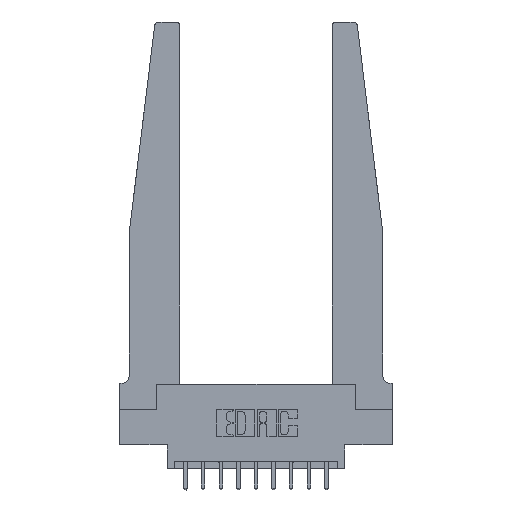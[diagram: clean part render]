
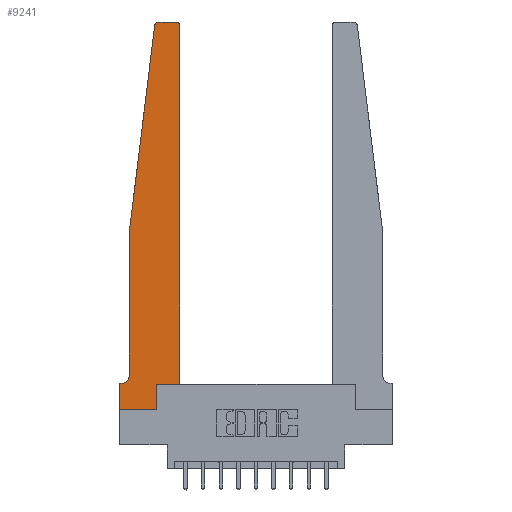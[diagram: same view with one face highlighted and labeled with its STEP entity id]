
A CAD part, top view. The second image highlights one B-rep face of the part: STEP entity #9241.
In plain terms, the highlighted planar face has unit normal (0, 0, 1).
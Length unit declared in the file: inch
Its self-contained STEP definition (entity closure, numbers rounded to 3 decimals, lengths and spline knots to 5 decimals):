
#208 = DIRECTION ( 'NONE',  ( -0.122, -0.992, 0. ) ) ;
#291 = DIRECTION ( 'NONE',  ( 0., 1., 0. ) ) ;
#334 = AXIS2_PLACEMENT_3D ( 'NONE', #9579, #2509, #10757 ) ;
#361 = VERTEX_POINT ( 'NONE', #12721 ) ;
#420 = CARTESIAN_POINT ( 'NONE',  ( 0.25, 2.75, 0.37 ) ) ;
#540 = CARTESIAN_POINT ( 'NONE',  ( 0.425, 0.18, 0.37 ) ) ;
#568 = EDGE_CURVE ( 'NONE', #1112, #13884, #9893, .T. ) ;
#876 = DIRECTION ( 'NONE',  ( 0., 0., 1. ) ) ;
#1070 = DIRECTION ( 'NONE',  ( -1., 0., 0. ) ) ;
#1112 = VERTEX_POINT ( 'NONE', #11998 ) ;
#1136 = CARTESIAN_POINT ( 'NONE',  ( 0., 0.1875, 0.37 ) ) ;
#1225 = EDGE_CURVE ( 'NONE', #2982, #15082, #8780, .T. ) ;
#1309 = ORIENTED_EDGE ( 'NONE', *, *, #10049, .T. ) ;
#1321 = CARTESIAN_POINT ( 'NONE',  ( 0.065, 0.1875, 0.37 ) ) ;
#1720 = AXIS2_PLACEMENT_3D ( 'NONE', #7896, #876, #9090 ) ;
#1835 = ORIENTED_EDGE ( 'NONE', *, *, #5461, .T. ) ;
#2044 = EDGE_CURVE ( 'NONE', #4084, #5762, #12457, .T. ) ;
#2156 = LINE ( 'NONE', #9585, #14345 ) ;
#2312 = CARTESIAN_POINT ( 'NONE',  ( 0.065, 1.25, 0.37 ) ) ;
#2509 = DIRECTION ( 'NONE',  ( 0., 0., 1. ) ) ;
#2982 = VERTEX_POINT ( 'NONE', #12450 ) ;
#3223 = CARTESIAN_POINT ( 'NONE',  ( 0.425, 0.18, 0.37 ) ) ;
#3772 = VECTOR ( 'NONE', #208, 39.37008 ) ;
#3892 = CIRCLE ( 'NONE', #6636, 0.03 ) ;
#4011 = AXIS2_PLACEMENT_3D ( 'NONE', #15167, #8103, #1070 ) ;
#4020 = VECTOR ( 'NONE', #7918, 39.37008 ) ;
#4084 = VERTEX_POINT ( 'NONE', #8564 ) ;
#4137 = CARTESIAN_POINT ( 'NONE',  ( 0.2605, 0.18, 0.37 ) ) ;
#4456 = ORIENTED_EDGE ( 'NONE', *, *, #14058, .T. ) ;
#4573 = EDGE_CURVE ( 'NONE', #7315, #1112, #5723, .T. ) ;
#4745 = ORIENTED_EDGE ( 'NONE', *, *, #12419, .T. ) ;
#5059 = EDGE_LOOP ( 'NONE', ( #5064, #1309, #12582, #4745, #6659, #11967, #1835, #11521, #14530, #4456, #9720, #8809 ) ) ;
#5064 = ORIENTED_EDGE ( 'NONE', *, *, #568, .T. ) ;
#5240 = EDGE_CURVE ( 'NONE', #5762, #14601, #10142, .T. ) ;
#5427 = CARTESIAN_POINT ( 'NONE',  ( 0.425, 2.72, 0.37 ) ) ;
#5461 = EDGE_CURVE ( 'NONE', #14601, #2982, #7173, .T. ) ;
#5523 = PLANE ( 'NONE',  #1720 ) ;
#5723 = CIRCLE ( 'NONE', #334, 0.03 ) ;
#5762 = VERTEX_POINT ( 'NONE', #8244 ) ;
#6111 = CARTESIAN_POINT ( 'NONE',  ( 0.425, 0.18, 0.37 ) ) ;
#6636 = AXIS2_PLACEMENT_3D ( 'NONE', #6956, #15228, #8160 ) ;
#6659 = ORIENTED_EDGE ( 'NONE', *, *, #2044, .T. ) ;
#6783 = DIRECTION ( 'NONE',  ( -1., 0., 0. ) ) ;
#6956 = CARTESIAN_POINT ( 'NONE',  ( 0.27653, 2.72, 0.37 ) ) ;
#6998 = VECTOR ( 'NONE', #9661, 39.37008 ) ;
#7074 = EDGE_CURVE ( 'NONE', #361, #13538, #13182, .T. ) ;
#7135 = LINE ( 'NONE', #3223, #4020 ) ;
#7173 = LINE ( 'NONE', #8831, #13088 ) ;
#7315 = VERTEX_POINT ( 'NONE', #5427 ) ;
#7667 = CARTESIAN_POINT ( 'NONE',  ( 0.27653, 2.75, 0.37 ) ) ;
#7896 = CARTESIAN_POINT ( 'NONE',  ( 0., 0.1875, 0.37 ) ) ;
#7918 = DIRECTION ( 'NONE',  ( 1., 0., 0. ) ) ;
#8030 = VECTOR ( 'NONE', #8179, 39.37008 ) ;
#8103 = DIRECTION ( 'NONE',  ( 0., 0., -1. ) ) ;
#8160 = DIRECTION ( 'NONE',  ( 1., 0., 0. ) ) ;
#8179 = DIRECTION ( 'NONE',  ( 1., 0., 0. ) ) ;
#8244 = CARTESIAN_POINT ( 'NONE',  ( 0.015, 0.1875, 0.37 ) ) ;
#8564 = CARTESIAN_POINT ( 'NONE',  ( 0.065, 0.2375, 0.37 ) ) ;
#8780 = LINE ( 'NONE', #11184, #8030 ) ;
#8809 = ORIENTED_EDGE ( 'NONE', *, *, #4573, .T. ) ;
#8831 = CARTESIAN_POINT ( 'NONE',  ( 0., 0., 0.37 ) ) ;
#8839 = VECTOR ( 'NONE', #291, 39.37008 ) ;
#9090 = DIRECTION ( 'NONE',  ( 1., 0., 0. ) ) ;
#9211 = LINE ( 'NONE', #6111, #8839 ) ;
#9241 = ADVANCED_FACE ( 'NONE', ( #12224 ), #5523, .T. ) ;
#9372 = CARTESIAN_POINT ( 'NONE',  ( 0.2605, 0.18, 0.37 ) ) ;
#9531 = VECTOR ( 'NONE', #6783, 39.37008 ) ;
#9579 = CARTESIAN_POINT ( 'NONE',  ( 0.395, 2.72, 0.37 ) ) ;
#9585 = CARTESIAN_POINT ( 'NONE',  ( 0.065, 1.25, 0.37 ) ) ;
#9661 = DIRECTION ( 'NONE',  ( -1., 0., 0. ) ) ;
#9720 = ORIENTED_EDGE ( 'NONE', *, *, #13704, .T. ) ;
#9763 = EDGE_CURVE ( 'NONE', #15082, #14181, #13858, .T. ) ;
#9893 = LINE ( 'NONE', #420, #9531 ) ;
#9998 = DIRECTION ( 'NONE',  ( 0., -1., 0. ) ) ;
#10049 = EDGE_CURVE ( 'NONE', #13884, #361, #3892, .T. ) ;
#10108 = CARTESIAN_POINT ( 'NONE',  ( 0.2605, 0., 0.37 ) ) ;
#10142 = LINE ( 'NONE', #1321, #6998 ) ;
#10720 = VECTOR ( 'NONE', #11186, 39.37008 ) ;
#10757 = DIRECTION ( 'NONE',  ( 1., 0., 0. ) ) ;
#10760 = DIRECTION ( 'NONE',  ( 0., -1., 0. ) ) ;
#11024 = VERTEX_POINT ( 'NONE', #540 ) ;
#11184 = CARTESIAN_POINT ( 'NONE',  ( 0., 0., 0.37 ) ) ;
#11186 = DIRECTION ( 'NONE',  ( 0., 1., 0. ) ) ;
#11521 = ORIENTED_EDGE ( 'NONE', *, *, #1225, .T. ) ;
#11967 = ORIENTED_EDGE ( 'NONE', *, *, #5240, .T. ) ;
#11998 = CARTESIAN_POINT ( 'NONE',  ( 0.395, 2.75, 0.37 ) ) ;
#12224 = FACE_OUTER_BOUND ( 'NONE', #5059, .T. ) ;
#12419 = EDGE_CURVE ( 'NONE', #13538, #4084, #2156, .T. ) ;
#12450 = CARTESIAN_POINT ( 'NONE',  ( 0., 0., 0.37 ) ) ;
#12457 = CIRCLE ( 'NONE', #4011, 0.05 ) ;
#12582 = ORIENTED_EDGE ( 'NONE', *, *, #7074, .T. ) ;
#12721 = CARTESIAN_POINT ( 'NONE',  ( 0.24675, 2.72367, 0.37 ) ) ;
#13088 = VECTOR ( 'NONE', #9998, 39.37008 ) ;
#13182 = LINE ( 'NONE', #14308, #3772 ) ;
#13538 = VERTEX_POINT ( 'NONE', #2312 ) ;
#13704 = EDGE_CURVE ( 'NONE', #11024, #7315, #9211, .T. ) ;
#13858 = LINE ( 'NONE', #4137, #10720 ) ;
#13884 = VERTEX_POINT ( 'NONE', #7667 ) ;
#14058 = EDGE_CURVE ( 'NONE', #14181, #11024, #7135, .T. ) ;
#14181 = VERTEX_POINT ( 'NONE', #9372 ) ;
#14308 = CARTESIAN_POINT ( 'NONE',  ( 0.065, 1.25, 0.37 ) ) ;
#14345 = VECTOR ( 'NONE', #10760, 39.37008 ) ;
#14530 = ORIENTED_EDGE ( 'NONE', *, *, #9763, .T. ) ;
#14601 = VERTEX_POINT ( 'NONE', #1136 ) ;
#15082 = VERTEX_POINT ( 'NONE', #10108 ) ;
#15167 = CARTESIAN_POINT ( 'NONE',  ( 0.015, 0.2375, 0.37 ) ) ;
#15228 = DIRECTION ( 'NONE',  ( 0., 0., 1. ) ) ;
